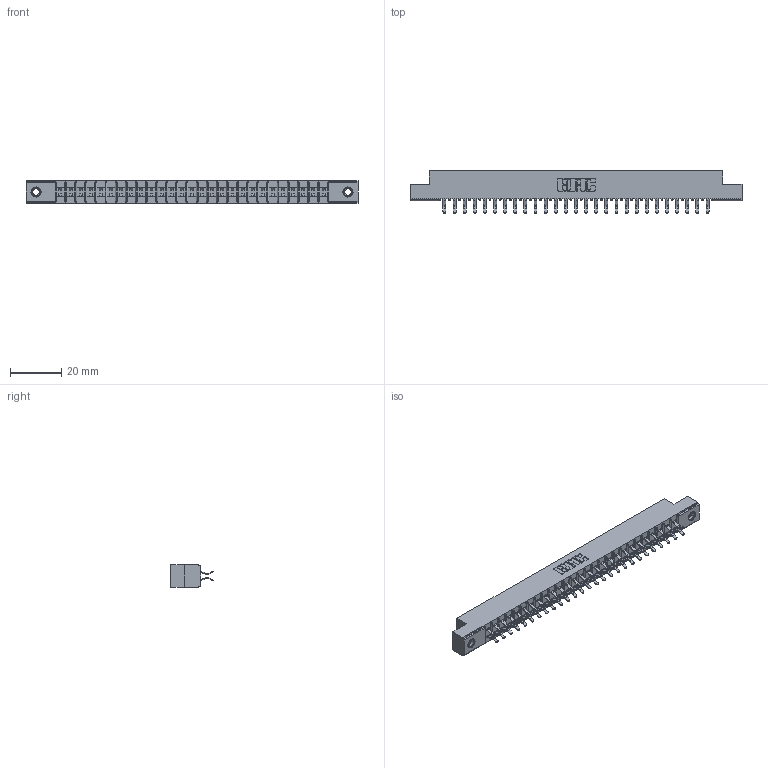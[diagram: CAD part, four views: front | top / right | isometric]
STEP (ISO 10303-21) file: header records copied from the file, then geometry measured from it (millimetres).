
FILE_DESCRIPTION (( 'STEP AP203' ), '1' );
FILE_NAME ('355-054-556-207.STEP', '2019-09-11T17:19:32', ( '' ), ( '' ), 'SwSTEP 2.0', 'SolidWorks 2016', '' );
FILE_SCHEMA (( 'CONFIG_CONTROL_DESIGN' ));
Length unit declared in the file: inch
Products named in the file (4): 305 Part_.156 Dia; 345-250-001_345-250-005-103; 305-290-001_556; 355-054-556-207
Assembly tree (57 placements, depth 2):
  355-054-556-207
    305 Part_.156 Dia
    305-290-001_556  x54
    345-250-001_345-250-005-103  x2
Bounding box: 130 x 16.64 x 8.71 mm (x, y, z)
Volume: 8119.7 mm3; surface area: 15697.7 mm2
Topology: 57 solids, 57 shells, 3200 faces, 9173 edges, 5962 vertices
Faces by surface type: plane 1774, cylinder 1302, sphere 108, cone 12, torus 4
Entity records: 32467 total; most frequent: CARTESIAN_POINT 5358, ORIENTED_EDGE 5310, DIRECTION 5209, EDGE_CURVE 2655, VECTOR 2123, LINE 2123, VERTEX_POINT 1692, AXIS2_PLACEMENT_3D 1543
